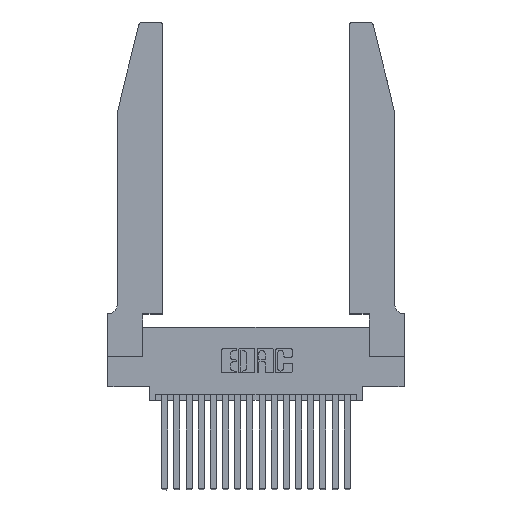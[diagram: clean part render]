
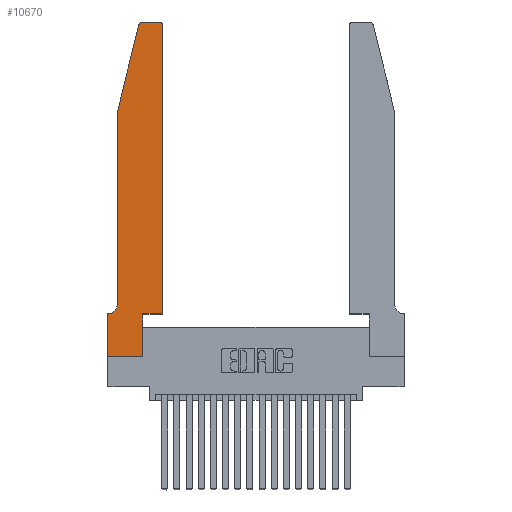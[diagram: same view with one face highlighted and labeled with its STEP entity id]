
A CAD part, top view. The second image highlights one B-rep face of the part: STEP entity #10670.
In plain terms, the highlighted planar face has unit normal (0, 0, 1).
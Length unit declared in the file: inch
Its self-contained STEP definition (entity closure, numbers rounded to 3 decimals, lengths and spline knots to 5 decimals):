
#135 = AXIS2_PLACEMENT_3D ( 'NONE', #20687, #11061, #12684 ) ;
#214 = DIRECTION ( 'NONE',  ( 0., -1., 0. ) ) ;
#311 = EDGE_CURVE ( 'NONE', #16349, #8537, #7692, .T. ) ;
#355 = CARTESIAN_POINT ( 'NONE',  ( 0.4505, 0.35, 0.37 ) ) ;
#765 = CARTESIAN_POINT ( 'NONE',  ( 0., 0., 0.37 ) ) ;
#1669 = CARTESIAN_POINT ( 'NONE',  ( 0.0755, 2., 0.37 ) ) ;
#1927 = CARTESIAN_POINT ( 'NONE',  ( 0., 0., 0.37 ) ) ;
#1941 = VERTEX_POINT ( 'NONE', #9356 ) ;
#2054 = VERTEX_POINT ( 'NONE', #11288 ) ;
#2285 = CIRCLE ( 'NONE', #135, 0.03 ) ;
#2306 = VECTOR ( 'NONE', #20699, 39.37008 ) ;
#2497 = FACE_OUTER_BOUND ( 'NONE', #9930, .T. ) ;
#2559 = CARTESIAN_POINT ( 'NONE',  ( 0., 0.35, 0.37 ) ) ;
#2564 = LINE ( 'NONE', #17625, #2306 ) ;
#2621 = VECTOR ( 'NONE', #9792, 39.37008 ) ;
#2625 = VECTOR ( 'NONE', #6778, 39.37008 ) ;
#3112 = CARTESIAN_POINT ( 'NONE',  ( 0.0755, 2., 0.37 ) ) ;
#3134 = DIRECTION ( 'NONE',  ( 0., 0., 1. ) ) ;
#3143 = ORIENTED_EDGE ( 'NONE', *, *, #10003, .T. ) ;
#3264 = DIRECTION ( 'NONE',  ( -0.239, -0.971, 0. ) ) ;
#3685 = LINE ( 'NONE', #1927, #11398 ) ;
#4055 = LINE ( 'NONE', #17778, #10286 ) ;
#4646 = CIRCLE ( 'NONE', #13218, 0.07 ) ;
#4678 = DIRECTION ( 'NONE',  ( 1., 0., 0. ) ) ;
#4715 = DIRECTION ( 'NONE',  ( 0., 0., -1. ) ) ;
#4831 = VERTEX_POINT ( 'NONE', #15798 ) ;
#5236 = DIRECTION ( 'NONE',  ( 0., 1., 0. ) ) ;
#5898 = LINE ( 'NONE', #355, #13360 ) ;
#6001 = ORIENTED_EDGE ( 'NONE', *, *, #20484, .T. ) ;
#6028 = CIRCLE ( 'NONE', #14707, 0.03 ) ;
#6301 = DIRECTION ( 'NONE',  ( -1., 0., 0. ) ) ;
#6774 = VERTEX_POINT ( 'NONE', #18356 ) ;
#6778 = DIRECTION ( 'NONE',  ( 0., 1., 0. ) ) ;
#7349 = LINE ( 'NONE', #9762, #2625 ) ;
#7638 = LINE ( 'NONE', #20343, #9627 ) ;
#7692 = LINE ( 'NONE', #3112, #19725 ) ;
#8033 = DIRECTION ( 'NONE',  ( 0., -1., 0. ) ) ;
#8210 = LINE ( 'NONE', #1669, #10178 ) ;
#8277 = EDGE_CURVE ( 'NONE', #2054, #4831, #4646, .T. ) ;
#8379 = ORIENTED_EDGE ( 'NONE', *, *, #13406, .T. ) ;
#8537 = VERTEX_POINT ( 'NONE', #20081 ) ;
#8634 = CARTESIAN_POINT ( 'NONE',  ( 0.25487, 2.72718, 0.37 ) ) ;
#8694 = DIRECTION ( 'NONE',  ( 1., 0., 0. ) ) ;
#9356 = CARTESIAN_POINT ( 'NONE',  ( 0.4505, 2.72, 0.37 ) ) ;
#9622 = DIRECTION ( 'NONE',  ( -1., 0., 0. ) ) ;
#9627 = VECTOR ( 'NONE', #14973, 39.37008 ) ;
#9657 = EDGE_CURVE ( 'NONE', #19606, #16396, #19402, .T. ) ;
#9733 = ORIENTED_EDGE ( 'NONE', *, *, #15495, .T. ) ;
#9762 = CARTESIAN_POINT ( 'NONE',  ( 0.2865, 0.35, 0.37 ) ) ;
#9792 = DIRECTION ( 'NONE',  ( 1., 0., 0. ) ) ;
#9930 = EDGE_LOOP ( 'NONE', ( #8379, #20746, #19269, #19975, #18564, #9733, #13977, #19778, #18837, #6001, #15374, #3143 ) ) ;
#10003 = EDGE_CURVE ( 'NONE', #1941, #18323, #6028, .T. ) ;
#10178 = VECTOR ( 'NONE', #8033, 39.37008 ) ;
#10286 = VECTOR ( 'NONE', #9622, 39.37008 ) ;
#10670 = ADVANCED_FACE ( 'NONE', ( #2497 ), #12025, .T. ) ;
#11061 = DIRECTION ( 'NONE',  ( 0., 0., 1. ) ) ;
#11288 = CARTESIAN_POINT ( 'NONE',  ( 0.0755, 0.42, 0.37 ) ) ;
#11291 = CARTESIAN_POINT ( 'NONE',  ( 0.4205, 2.75, 0.37 ) ) ;
#11327 = VERTEX_POINT ( 'NONE', #12020 ) ;
#11398 = VECTOR ( 'NONE', #214, 39.37008 ) ;
#11809 = DIRECTION ( 'NONE',  ( 0., 0., 1. ) ) ;
#12020 = CARTESIAN_POINT ( 'NONE',  ( 0.284, 2.75, 0.37 ) ) ;
#12025 = PLANE ( 'NONE',  #14439 ) ;
#12684 = DIRECTION ( 'NONE',  ( 1., 0., 0. ) ) ;
#13125 = CARTESIAN_POINT ( 'NONE',  ( 0.2865, 0.35, 0.37 ) ) ;
#13218 = AXIS2_PLACEMENT_3D ( 'NONE', #17791, #4715, #6301 ) ;
#13288 = CARTESIAN_POINT ( 'NONE',  ( 0., 0., 0.37 ) ) ;
#13360 = VECTOR ( 'NONE', #5236, 39.37008 ) ;
#13406 = EDGE_CURVE ( 'NONE', #18323, #11327, #7638, .T. ) ;
#13677 = EDGE_CURVE ( 'NONE', #16629, #1941, #5898, .T. ) ;
#13954 = EDGE_CURVE ( 'NONE', #16396, #17454, #7349, .T. ) ;
#13977 = ORIENTED_EDGE ( 'NONE', *, *, #17818, .T. ) ;
#14408 = CARTESIAN_POINT ( 'NONE',  ( 0.4505, 0.35, 0.37 ) ) ;
#14439 = AXIS2_PLACEMENT_3D ( 'NONE', #2559, #11809, #8694 ) ;
#14707 = AXIS2_PLACEMENT_3D ( 'NONE', #17341, #3134, #4678 ) ;
#14973 = DIRECTION ( 'NONE',  ( -1., 0., 0. ) ) ;
#15374 = ORIENTED_EDGE ( 'NONE', *, *, #13677, .T. ) ;
#15495 = EDGE_CURVE ( 'NONE', #4831, #6774, #4055, .T. ) ;
#15798 = CARTESIAN_POINT ( 'NONE',  ( 0.0055, 0.35, 0.37 ) ) ;
#16030 = EDGE_CURVE ( 'NONE', #11327, #16349, #2285, .T. ) ;
#16349 = VERTEX_POINT ( 'NONE', #8634 ) ;
#16396 = VERTEX_POINT ( 'NONE', #16963 ) ;
#16629 = VERTEX_POINT ( 'NONE', #14408 ) ;
#16963 = CARTESIAN_POINT ( 'NONE',  ( 0.2865, 0., 0.37 ) ) ;
#17265 = EDGE_CURVE ( 'NONE', #8537, #2054, #8210, .T. ) ;
#17341 = CARTESIAN_POINT ( 'NONE',  ( 0.4205, 2.72, 0.37 ) ) ;
#17454 = VERTEX_POINT ( 'NONE', #13125 ) ;
#17625 = CARTESIAN_POINT ( 'NONE',  ( 0.4505, 0.35, 0.37 ) ) ;
#17778 = CARTESIAN_POINT ( 'NONE',  ( 0.0755, 0.35, 0.37 ) ) ;
#17791 = CARTESIAN_POINT ( 'NONE',  ( 0.0055, 0.42, 0.37 ) ) ;
#17818 = EDGE_CURVE ( 'NONE', #6774, #19606, #3685, .T. ) ;
#18323 = VERTEX_POINT ( 'NONE', #11291 ) ;
#18356 = CARTESIAN_POINT ( 'NONE',  ( 0., 0.35, 0.37 ) ) ;
#18564 = ORIENTED_EDGE ( 'NONE', *, *, #8277, .T. ) ;
#18837 = ORIENTED_EDGE ( 'NONE', *, *, #13954, .T. ) ;
#19269 = ORIENTED_EDGE ( 'NONE', *, *, #311, .T. ) ;
#19402 = LINE ( 'NONE', #13288, #2621 ) ;
#19606 = VERTEX_POINT ( 'NONE', #765 ) ;
#19725 = VECTOR ( 'NONE', #3264, 39.37008 ) ;
#19778 = ORIENTED_EDGE ( 'NONE', *, *, #9657, .T. ) ;
#19975 = ORIENTED_EDGE ( 'NONE', *, *, #17265, .T. ) ;
#20081 = CARTESIAN_POINT ( 'NONE',  ( 0.0755, 2., 0.37 ) ) ;
#20343 = CARTESIAN_POINT ( 'NONE',  ( 0.2605, 2.75, 0.37 ) ) ;
#20484 = EDGE_CURVE ( 'NONE', #17454, #16629, #2564, .T. ) ;
#20687 = CARTESIAN_POINT ( 'NONE',  ( 0.284, 2.72, 0.37 ) ) ;
#20699 = DIRECTION ( 'NONE',  ( 1., 0., 0. ) ) ;
#20746 = ORIENTED_EDGE ( 'NONE', *, *, #16030, .T. ) ;
